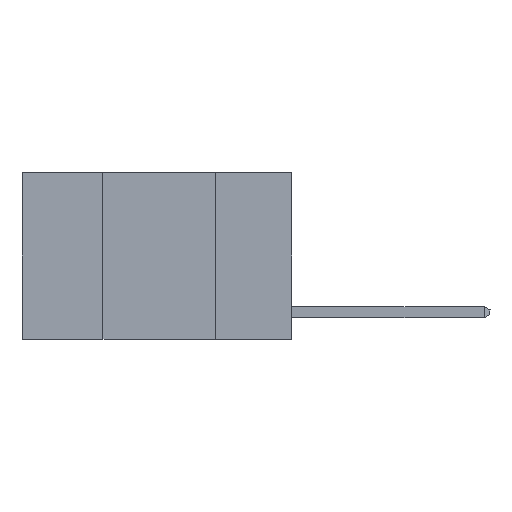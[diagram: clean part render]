
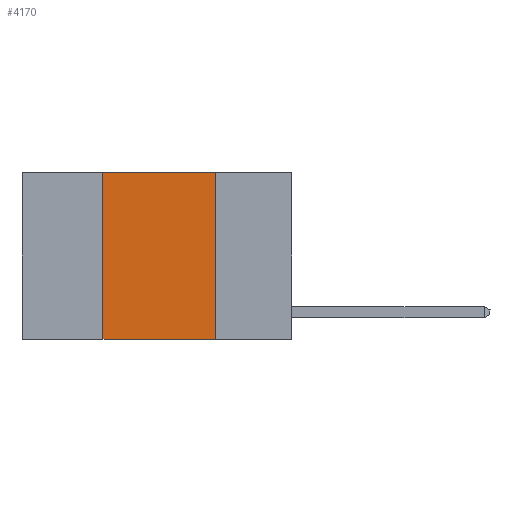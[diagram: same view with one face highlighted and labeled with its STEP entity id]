
A CAD part, left-side view. The second image highlights one B-rep face of the part: STEP entity #4170.
In plain terms, the highlighted planar face has unit normal (-1, 0, 0).
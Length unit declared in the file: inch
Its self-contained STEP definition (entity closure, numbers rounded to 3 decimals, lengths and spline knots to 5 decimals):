
#99 = FACE_OUTER_BOUND ( 'NONE', #11524, .T. ) ;
#246 = VECTOR ( 'NONE', #17134, 39.37008 ) ;
#1058 = CARTESIAN_POINT ( 'NONE',  ( 0., 0.6, 0. ) ) ;
#1543 = VECTOR ( 'NONE', #17603, 39.37008 ) ;
#2704 = DIRECTION ( 'NONE',  ( 1., 0., 0. ) ) ;
#2935 = CARTESIAN_POINT ( 'NONE',  ( 0., 0.6, -0.37 ) ) ;
#4170 = ADVANCED_FACE ( 'NONE', ( #99 ), #19879, .F. ) ;
#4926 = VERTEX_POINT ( 'NONE', #10233 ) ;
#5375 = ORIENTED_EDGE ( 'NONE', *, *, #19681, .F. ) ;
#5523 = VERTEX_POINT ( 'NONE', #17859 ) ;
#6696 = CARTESIAN_POINT ( 'NONE',  ( 0., 0.6, 0. ) ) ;
#7164 = DIRECTION ( 'NONE',  ( 0., 0., 1. ) ) ;
#8209 = DIRECTION ( 'NONE',  ( 0., 0., -1. ) ) ;
#9801 = AXIS2_PLACEMENT_3D ( 'NONE', #1058, #2704, #13829 ) ;
#10233 = CARTESIAN_POINT ( 'NONE',  ( 0., 0.17, -0.37 ) ) ;
#10275 = VERTEX_POINT ( 'NONE', #16262 ) ;
#10281 = CARTESIAN_POINT ( 'NONE',  ( 0., 0.42, 0. ) ) ;
#10522 = VECTOR ( 'NONE', #8209, 39.37008 ) ;
#11432 = EDGE_CURVE ( 'NONE', #5523, #4926, #18703, .T. ) ;
#11524 = EDGE_LOOP ( 'NONE', ( #16061, #5375, #14636, #12840 ) ) ;
#11931 = LINE ( 'NONE', #10281, #20034 ) ;
#12088 = CARTESIAN_POINT ( 'NONE',  ( 0., 0.42, -0.37 ) ) ;
#12840 = ORIENTED_EDGE ( 'NONE', *, *, #19479, .T. ) ;
#13024 = EDGE_CURVE ( 'NONE', #19981, #10275, #11931, .T. ) ;
#13748 = LINE ( 'NONE', #6696, #1543 ) ;
#13829 = DIRECTION ( 'NONE',  ( 0., 0., -1. ) ) ;
#14636 = ORIENTED_EDGE ( 'NONE', *, *, #13024, .F. ) ;
#15965 = CARTESIAN_POINT ( 'NONE',  ( 0., 0.17, 0. ) ) ;
#16061 = ORIENTED_EDGE ( 'NONE', *, *, #11432, .F. ) ;
#16262 = CARTESIAN_POINT ( 'NONE',  ( 0., 0.42, 0. ) ) ;
#17124 = LINE ( 'NONE', #2935, #246 ) ;
#17134 = DIRECTION ( 'NONE',  ( 0., -1., 0. ) ) ;
#17603 = DIRECTION ( 'NONE',  ( 0., -1., 0. ) ) ;
#17859 = CARTESIAN_POINT ( 'NONE',  ( 0., 0.17, 0. ) ) ;
#18703 = LINE ( 'NONE', #15965, #10522 ) ;
#19479 = EDGE_CURVE ( 'NONE', #19981, #4926, #17124, .T. ) ;
#19681 = EDGE_CURVE ( 'NONE', #10275, #5523, #13748, .T. ) ;
#19879 = PLANE ( 'NONE',  #9801 ) ;
#19981 = VERTEX_POINT ( 'NONE', #12088 ) ;
#20034 = VECTOR ( 'NONE', #7164, 39.37008 ) ;
